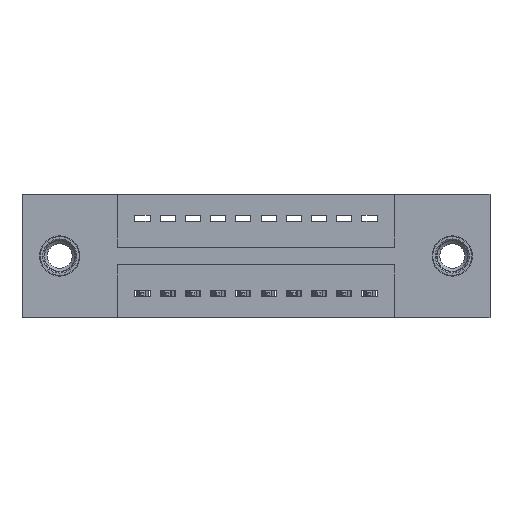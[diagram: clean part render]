
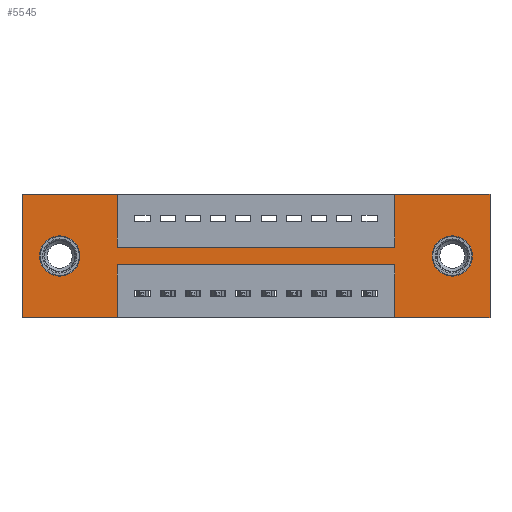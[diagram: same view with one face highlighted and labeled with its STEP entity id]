
A CAD part, front view. The second image highlights one B-rep face of the part: STEP entity #5545.
In plain terms, the highlighted planar face has unit normal (0, -1, 0).
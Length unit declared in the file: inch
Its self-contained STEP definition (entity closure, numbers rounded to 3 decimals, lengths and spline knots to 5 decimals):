
#44 = VERTEX_POINT ( 'NONE', #11258 ) ;
#140 = AXIS2_PLACEMENT_3D ( 'NONE', #5963, #1445, #5027 ) ;
#244 = CARTESIAN_POINT ( 'NONE',  ( 0., 0., -0.49 ) ) ;
#265 = DIRECTION ( 'NONE',  ( 0., 0., -1. ) ) ;
#350 = VERTEX_POINT ( 'NONE', #5158 ) ;
#513 = ORIENTED_EDGE ( 'NONE', *, *, #2381, .F. ) ;
#748 = EDGE_CURVE ( 'NONE', #6635, #4866, #9463, .T. ) ;
#761 = LINE ( 'NONE', #11456, #6310 ) ;
#818 = VERTEX_POINT ( 'NONE', #10607 ) ;
#879 = VECTOR ( 'NONE', #4537, 39.37008 ) ;
#1255 = FACE_BOUND ( 'NONE', #3279, .T. ) ;
#1287 = CIRCLE ( 'NONE', #11035, 0.08 ) ;
#1321 = ORIENTED_EDGE ( 'NONE', *, *, #6195, .T. ) ;
#1419 = CARTESIAN_POINT ( 'NONE',  ( 0., 0., 0. ) ) ;
#1444 = LINE ( 'NONE', #1671, #10571 ) ;
#1445 = DIRECTION ( 'NONE',  ( 0., 1., 0. ) ) ;
#1451 = CARTESIAN_POINT ( 'NONE',  ( 0., 0., 0. ) ) ;
#1556 = CARTESIAN_POINT ( 'NONE',  ( 0.3775, 0., -0.49 ) ) ;
#1671 = CARTESIAN_POINT ( 'NONE',  ( 0.3775, 0., -0.28 ) ) ;
#1761 = VECTOR ( 'NONE', #5684, 39.37008 ) ;
#1765 = VERTEX_POINT ( 'NONE', #1419 ) ;
#1843 = EDGE_CURVE ( 'NONE', #11055, #5350, #1287, .T. ) ;
#1940 = DIRECTION ( 'NONE',  ( 0., 0., -1. ) ) ;
#2015 = ORIENTED_EDGE ( 'NONE', *, *, #1843, .T. ) ;
#2044 = EDGE_CURVE ( 'NONE', #2711, #818, #3816, .T. ) ;
#2145 = CARTESIAN_POINT ( 'NONE',  ( 0., 0., 0. ) ) ;
#2198 = FACE_BOUND ( 'NONE', #2832, .T. ) ;
#2319 = CIRCLE ( 'NONE', #3736, 0.08 ) ;
#2332 = DIRECTION ( 'NONE',  ( 0., 0., 1. ) ) ;
#2338 = LINE ( 'NONE', #1451, #9541 ) ;
#2381 = EDGE_CURVE ( 'NONE', #8967, #350, #761, .T. ) ;
#2592 = DIRECTION ( 'NONE',  ( 0., -1., 0. ) ) ;
#2621 = VECTOR ( 'NONE', #7568, 39.37008 ) ;
#2663 = CARTESIAN_POINT ( 'NONE',  ( 0., 0., 0. ) ) ;
#2711 = VERTEX_POINT ( 'NONE', #1556 ) ;
#2804 = EDGE_CURVE ( 'NONE', #10573, #2711, #1444, .T. ) ;
#2832 = EDGE_LOOP ( 'NONE', ( #2015, #5705 ) ) ;
#3054 = DIRECTION ( 'NONE',  ( 0., 1., 0. ) ) ;
#3104 = CARTESIAN_POINT ( 'NONE',  ( 1.855, 0., 0. ) ) ;
#3165 = EDGE_CURVE ( 'NONE', #8262, #8140, #9462, .T. ) ;
#3274 = CARTESIAN_POINT ( 'NONE',  ( 0.1495, 0., -0.325 ) ) ;
#3279 = EDGE_LOOP ( 'NONE', ( #1321, #7645 ) ) ;
#3406 = VERTEX_POINT ( 'NONE', #7408 ) ;
#3591 = DIRECTION ( 'NONE',  ( 1., 0., 0. ) ) ;
#3708 = LINE ( 'NONE', #244, #9777 ) ;
#3736 = AXIS2_PLACEMENT_3D ( 'NONE', #9122, #3054, #265 ) ;
#3816 = LINE ( 'NONE', #4626, #7253 ) ;
#3903 = DIRECTION ( 'NONE',  ( -1., 0., 0. ) ) ;
#3916 = EDGE_CURVE ( 'NONE', #11045, #8967, #10977, .T. ) ;
#3920 = VECTOR ( 'NONE', #7567, 39.37008 ) ;
#4144 = LINE ( 'NONE', #4674, #1761 ) ;
#4191 = CARTESIAN_POINT ( 'NONE',  ( 0.1495, 0., -0.245 ) ) ;
#4227 = DIRECTION ( 'NONE',  ( 0., 0., 1. ) ) ;
#4327 = LINE ( 'NONE', #9225, #3920 ) ;
#4401 = CARTESIAN_POINT ( 'NONE',  ( 0., 0., -0.49 ) ) ;
#4537 = DIRECTION ( 'NONE',  ( 1., 0., 0. ) ) ;
#4572 = VERTEX_POINT ( 'NONE', #5324 ) ;
#4626 = CARTESIAN_POINT ( 'NONE',  ( 0., 0., -0.49 ) ) ;
#4674 = CARTESIAN_POINT ( 'NONE',  ( 0.3775, 0., -0.21 ) ) ;
#4774 = CARTESIAN_POINT ( 'NONE',  ( 1.4775, 0., -0.21 ) ) ;
#4852 = CARTESIAN_POINT ( 'NONE',  ( 0.3775, 0., -0.28 ) ) ;
#4866 = VERTEX_POINT ( 'NONE', #9576 ) ;
#4951 = CARTESIAN_POINT ( 'NONE',  ( 0.1495, 0., -0.165 ) ) ;
#5020 = CARTESIAN_POINT ( 'NONE',  ( 1.4775, 0., -0.28 ) ) ;
#5027 = DIRECTION ( 'NONE',  ( 0., 0., 1. ) ) ;
#5116 = ORIENTED_EDGE ( 'NONE', *, *, #5378, .F. ) ;
#5147 = VECTOR ( 'NONE', #5818, 39.37008 ) ;
#5158 = CARTESIAN_POINT ( 'NONE',  ( 1.855, 0., -0.49 ) ) ;
#5173 = EDGE_CURVE ( 'NONE', #1765, #4572, #5558, .T. ) ;
#5296 = CARTESIAN_POINT ( 'NONE',  ( 1.4775, 0., -0.21 ) ) ;
#5303 = EDGE_CURVE ( 'NONE', #818, #1765, #2338, .T. ) ;
#5324 = CARTESIAN_POINT ( 'NONE',  ( 0.3775, 0., 0. ) ) ;
#5350 = VERTEX_POINT ( 'NONE', #3274 ) ;
#5378 = EDGE_CURVE ( 'NONE', #44, #3406, #8991, .T. ) ;
#5467 = LINE ( 'NONE', #4774, #9334 ) ;
#5495 = CARTESIAN_POINT ( 'NONE',  ( 0.3775, 0., -0.21 ) ) ;
#5545 = ADVANCED_FACE ( 'NONE', ( #1255, #2198, #10103 ), #9668, .T. ) ;
#5558 = LINE ( 'NONE', #2145, #5147 ) ;
#5684 = DIRECTION ( 'NONE',  ( 0., 0., -1. ) ) ;
#5705 = ORIENTED_EDGE ( 'NONE', *, *, #10775, .T. ) ;
#5818 = DIRECTION ( 'NONE',  ( 1., 0., 0. ) ) ;
#5963 = CARTESIAN_POINT ( 'NONE',  ( 0.1495, 0., -0.245 ) ) ;
#6195 = EDGE_CURVE ( 'NONE', #4866, #6635, #2319, .T. ) ;
#6223 = CARTESIAN_POINT ( 'NONE',  ( 1.4775, 0., 0. ) ) ;
#6271 = VECTOR ( 'NONE', #3591, 39.37008 ) ;
#6310 = VECTOR ( 'NONE', #7080, 39.37008 ) ;
#6361 = ORIENTED_EDGE ( 'NONE', *, *, #11114, .F. ) ;
#6635 = VERTEX_POINT ( 'NONE', #7088 ) ;
#6673 = ORIENTED_EDGE ( 'NONE', *, *, #6835, .F. ) ;
#6779 = EDGE_CURVE ( 'NONE', #350, #44, #3708, .T. ) ;
#6835 = EDGE_CURVE ( 'NONE', #4572, #8262, #4144, .T. ) ;
#6898 = ORIENTED_EDGE ( 'NONE', *, *, #5173, .F. ) ;
#7080 = DIRECTION ( 'NONE',  ( 0., 0., -1. ) ) ;
#7088 = CARTESIAN_POINT ( 'NONE',  ( 1.7055, 0., -0.325 ) ) ;
#7253 = VECTOR ( 'NONE', #9789, 39.37008 ) ;
#7342 = CARTESIAN_POINT ( 'NONE',  ( 1.7055, 0., -0.245 ) ) ;
#7408 = CARTESIAN_POINT ( 'NONE',  ( 1.4775, 0., -0.28 ) ) ;
#7548 = ORIENTED_EDGE ( 'NONE', *, *, #2044, .F. ) ;
#7567 = DIRECTION ( 'NONE',  ( -1., 0., 0. ) ) ;
#7568 = DIRECTION ( 'NONE',  ( 0., 0., 1. ) ) ;
#7645 = ORIENTED_EDGE ( 'NONE', *, *, #748, .T. ) ;
#8140 = VERTEX_POINT ( 'NONE', #5296 ) ;
#8262 = VERTEX_POINT ( 'NONE', #5495 ) ;
#8793 = DIRECTION ( 'NONE',  ( 0., 0., -1. ) ) ;
#8931 = CARTESIAN_POINT ( 'NONE',  ( 0.3775, 0., -0.21 ) ) ;
#8947 = EDGE_LOOP ( 'NONE', ( #11181, #10904, #6673, #6898, #9437, #7548, #10321, #6361, #5116, #9510, #513, #11116 ) ) ;
#8967 = VERTEX_POINT ( 'NONE', #3104 ) ;
#8991 = LINE ( 'NONE', #5020, #2621 ) ;
#9019 = CIRCLE ( 'NONE', #140, 0.08 ) ;
#9122 = CARTESIAN_POINT ( 'NONE',  ( 1.7055, 0., -0.245 ) ) ;
#9225 = CARTESIAN_POINT ( 'NONE',  ( 0.3775, 0., -0.28 ) ) ;
#9334 = VECTOR ( 'NONE', #9411, 39.37008 ) ;
#9411 = DIRECTION ( 'NONE',  ( 0., 0., 1. ) ) ;
#9437 = ORIENTED_EDGE ( 'NONE', *, *, #5303, .F. ) ;
#9462 = LINE ( 'NONE', #8931, #879 ) ;
#9463 = CIRCLE ( 'NONE', #11314, 0.08 ) ;
#9510 = ORIENTED_EDGE ( 'NONE', *, *, #6779, .F. ) ;
#9541 = VECTOR ( 'NONE', #2332, 39.37008 ) ;
#9554 = AXIS2_PLACEMENT_3D ( 'NONE', #4401, #2592, #8793 ) ;
#9576 = CARTESIAN_POINT ( 'NONE',  ( 1.7055, 0., -0.165 ) ) ;
#9668 = PLANE ( 'NONE',  #9554 ) ;
#9691 = EDGE_CURVE ( 'NONE', #8140, #11045, #5467, .T. ) ;
#9777 = VECTOR ( 'NONE', #3903, 39.37008 ) ;
#9789 = DIRECTION ( 'NONE',  ( -1., 0., 0. ) ) ;
#10103 = FACE_OUTER_BOUND ( 'NONE', #8947, .T. ) ;
#10321 = ORIENTED_EDGE ( 'NONE', *, *, #2804, .F. ) ;
#10571 = VECTOR ( 'NONE', #10608, 39.37008 ) ;
#10573 = VERTEX_POINT ( 'NONE', #4852 ) ;
#10607 = CARTESIAN_POINT ( 'NONE',  ( 0., 0., -0.49 ) ) ;
#10608 = DIRECTION ( 'NONE',  ( 0., 0., -1. ) ) ;
#10775 = EDGE_CURVE ( 'NONE', #5350, #11055, #9019, .T. ) ;
#10778 = DIRECTION ( 'NONE',  ( 0., 1., 0. ) ) ;
#10904 = ORIENTED_EDGE ( 'NONE', *, *, #3165, .F. ) ;
#10977 = LINE ( 'NONE', #2663, #6271 ) ;
#11035 = AXIS2_PLACEMENT_3D ( 'NONE', #4191, #11246, #4227 ) ;
#11045 = VERTEX_POINT ( 'NONE', #6223 ) ;
#11055 = VERTEX_POINT ( 'NONE', #4951 ) ;
#11114 = EDGE_CURVE ( 'NONE', #3406, #10573, #4327, .T. ) ;
#11116 = ORIENTED_EDGE ( 'NONE', *, *, #3916, .F. ) ;
#11181 = ORIENTED_EDGE ( 'NONE', *, *, #9691, .F. ) ;
#11246 = DIRECTION ( 'NONE',  ( 0., 1., 0. ) ) ;
#11258 = CARTESIAN_POINT ( 'NONE',  ( 1.4775, 0., -0.49 ) ) ;
#11314 = AXIS2_PLACEMENT_3D ( 'NONE', #7342, #10778, #1940 ) ;
#11456 = CARTESIAN_POINT ( 'NONE',  ( 1.855, 0., 0. ) ) ;
